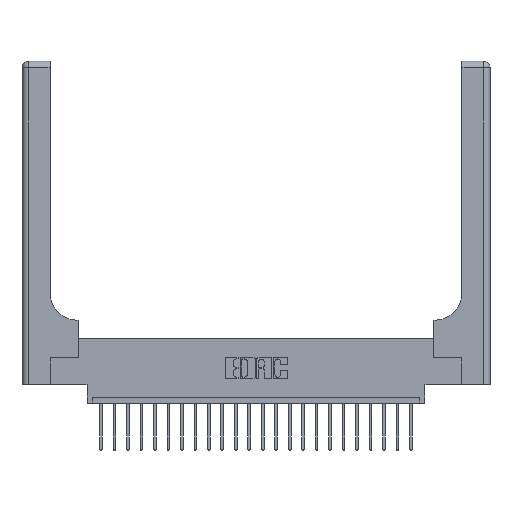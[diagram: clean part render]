
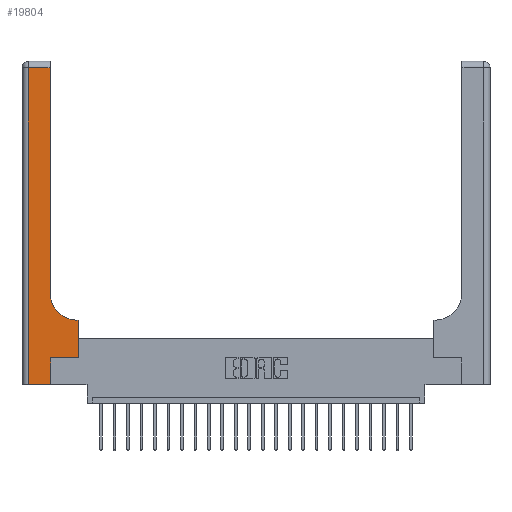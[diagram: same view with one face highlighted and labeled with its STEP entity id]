
A CAD part, top view. The second image highlights one B-rep face of the part: STEP entity #19804.
In plain terms, the highlighted planar face has unit normal (0, 0, 1).
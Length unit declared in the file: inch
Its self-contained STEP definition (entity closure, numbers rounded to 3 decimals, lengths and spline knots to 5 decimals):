
#420 = CARTESIAN_POINT ( 'NONE',  ( 0.528, 0.25, 0.37 ) ) ;
#828 = VERTEX_POINT ( 'NONE', #8844 ) ;
#972 = DIRECTION ( 'NONE',  ( 0., 1., 0. ) ) ;
#977 = DIRECTION ( 'NONE',  ( 1., 0., 0. ) ) ;
#1270 = VECTOR ( 'NONE', #19749, 39.37008 ) ;
#1829 = VERTEX_POINT ( 'NONE', #14032 ) ;
#2189 = CARTESIAN_POINT ( 'NONE',  ( 0.51, 0.85, 0.37 ) ) ;
#2507 = EDGE_CURVE ( 'NONE', #828, #2738, #18523, .T. ) ;
#2738 = VERTEX_POINT ( 'NONE', #7645 ) ;
#3773 = EDGE_CURVE ( 'NONE', #9672, #4569, #16127, .T. ) ;
#3791 = VERTEX_POINT ( 'NONE', #9495 ) ;
#4000 = ORIENTED_EDGE ( 'NONE', *, *, #4153, .T. ) ;
#4153 = EDGE_CURVE ( 'NONE', #3791, #9672, #22657, .T. ) ;
#4207 = ORIENTED_EDGE ( 'NONE', *, *, #3773, .T. ) ;
#4343 = ORIENTED_EDGE ( 'NONE', *, *, #5418, .T. ) ;
#4566 = LINE ( 'NONE', #11386, #14662 ) ;
#4569 = VERTEX_POINT ( 'NONE', #6475 ) ;
#4622 = DIRECTION ( 'NONE',  ( -1., 0., 0. ) ) ;
#5418 = EDGE_CURVE ( 'NONE', #5621, #3791, #22631, .T. ) ;
#5442 = VECTOR ( 'NONE', #972, 39.37008 ) ;
#5505 = DIRECTION ( 'NONE',  ( 1., 0., 0. ) ) ;
#5520 = CARTESIAN_POINT ( 'NONE',  ( 0., 0., 0.37 ) ) ;
#5621 = VERTEX_POINT ( 'NONE', #7108 ) ;
#5822 = VERTEX_POINT ( 'NONE', #21941 ) ;
#5887 = CARTESIAN_POINT ( 'NONE',  ( 0.26, 0.6, 0.37 ) ) ;
#5988 = VECTOR ( 'NONE', #21888, 39.37008 ) ;
#6475 = CARTESIAN_POINT ( 'NONE',  ( 0.06, 0., 0.37 ) ) ;
#6744 = CARTESIAN_POINT ( 'NONE',  ( 0., 3., 0.37 ) ) ;
#6857 = ORIENTED_EDGE ( 'NONE', *, *, #12726, .T. ) ;
#7020 = EDGE_LOOP ( 'NONE', ( #4343, #4000, #4207, #9555, #13726, #6857, #16717, #9166, #11224 ) ) ;
#7108 = CARTESIAN_POINT ( 'NONE',  ( 0.26, 0.85, 0.37 ) ) ;
#7361 = EDGE_CURVE ( 'NONE', #1829, #5621, #21461, .T. ) ;
#7645 = CARTESIAN_POINT ( 'NONE',  ( 0.265, 0.25, 0.37 ) ) ;
#7953 = CARTESIAN_POINT ( 'NONE',  ( 0.26, 3., 0.37 ) ) ;
#8422 = FACE_OUTER_BOUND ( 'NONE', #7020, .T. ) ;
#8748 = PLANE ( 'NONE',  #17469 ) ;
#8844 = CARTESIAN_POINT ( 'NONE',  ( 0.265, 0., 0.37 ) ) ;
#9166 = ORIENTED_EDGE ( 'NONE', *, *, #11754, .T. ) ;
#9495 = CARTESIAN_POINT ( 'NONE',  ( 0.26, 2.94, 0.37 ) ) ;
#9555 = ORIENTED_EDGE ( 'NONE', *, *, #21003, .T. ) ;
#9672 = VERTEX_POINT ( 'NONE', #21417 ) ;
#10110 = VECTOR ( 'NONE', #4622, 39.37008 ) ;
#10809 = LINE ( 'NONE', #5520, #18447 ) ;
#11224 = ORIENTED_EDGE ( 'NONE', *, *, #7361, .T. ) ;
#11386 = CARTESIAN_POINT ( 'NONE',  ( 0.265, 0.25, 0.37 ) ) ;
#11754 = EDGE_CURVE ( 'NONE', #5822, #1829, #20386, .T. ) ;
#12726 = EDGE_CURVE ( 'NONE', #2738, #22602, #4566, .T. ) ;
#13151 = CARTESIAN_POINT ( 'NONE',  ( 0.528, 0.25, 0.37 ) ) ;
#13726 = ORIENTED_EDGE ( 'NONE', *, *, #2507, .T. ) ;
#14032 = CARTESIAN_POINT ( 'NONE',  ( 0.51, 0.6, 0.37 ) ) ;
#14662 = VECTOR ( 'NONE', #977, 39.37008 ) ;
#14753 = CARTESIAN_POINT ( 'NONE',  ( 0.06, 3., 0.37 ) ) ;
#15049 = CARTESIAN_POINT ( 'NONE',  ( 0.265, 0., 0.37 ) ) ;
#15133 = CARTESIAN_POINT ( 'NONE',  ( 0., 2.94, 0.37 ) ) ;
#15660 = DIRECTION ( 'NONE',  ( 0., 0., -1. ) ) ;
#16127 = LINE ( 'NONE', #14753, #16907 ) ;
#16717 = ORIENTED_EDGE ( 'NONE', *, *, #19528, .T. ) ;
#16907 = VECTOR ( 'NONE', #19839, 39.37008 ) ;
#17140 = VECTOR ( 'NONE', #18329, 39.37008 ) ;
#17469 = AXIS2_PLACEMENT_3D ( 'NONE', #6744, #15660, #20595 ) ;
#17769 = DIRECTION ( 'NONE',  ( 1., 0., 0. ) ) ;
#18329 = DIRECTION ( 'NONE',  ( 0., 1., 0. ) ) ;
#18447 = VECTOR ( 'NONE', #17769, 39.37008 ) ;
#18523 = LINE ( 'NONE', #15049, #17140 ) ;
#19210 = AXIS2_PLACEMENT_3D ( 'NONE', #2189, #21357, #5505 ) ;
#19528 = EDGE_CURVE ( 'NONE', #22602, #5822, #20988, .T. ) ;
#19749 = DIRECTION ( 'NONE',  ( -1., 0., 0. ) ) ;
#19804 = ADVANCED_FACE ( 'NONE', ( #8422 ), #8748, .F. ) ;
#19839 = DIRECTION ( 'NONE',  ( 0., -1., 0. ) ) ;
#20386 = LINE ( 'NONE', #5887, #1270 ) ;
#20595 = DIRECTION ( 'NONE',  ( -1., 0., 0. ) ) ;
#20988 = LINE ( 'NONE', #13151, #5442 ) ;
#21003 = EDGE_CURVE ( 'NONE', #4569, #828, #10809, .T. ) ;
#21357 = DIRECTION ( 'NONE',  ( 0., 0., -1. ) ) ;
#21417 = CARTESIAN_POINT ( 'NONE',  ( 0.06, 2.94, 0.37 ) ) ;
#21461 = CIRCLE ( 'NONE', #19210, 0.25 ) ;
#21888 = DIRECTION ( 'NONE',  ( 0., 1., 0. ) ) ;
#21941 = CARTESIAN_POINT ( 'NONE',  ( 0.528, 0.6, 0.37 ) ) ;
#22602 = VERTEX_POINT ( 'NONE', #420 ) ;
#22631 = LINE ( 'NONE', #7953, #5988 ) ;
#22657 = LINE ( 'NONE', #15133, #10110 ) ;
